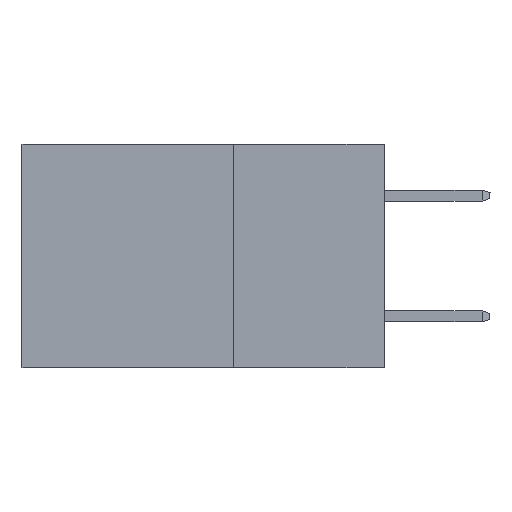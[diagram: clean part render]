
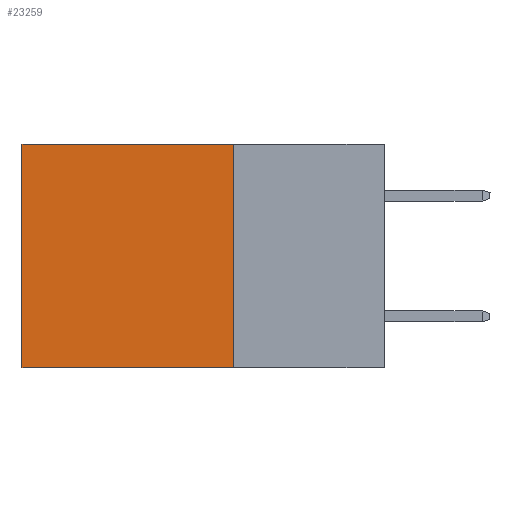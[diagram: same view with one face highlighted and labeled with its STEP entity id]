
A CAD part, left-side view. The second image highlights one B-rep face of the part: STEP entity #23259.
In plain terms, the highlighted planar face has unit normal (-1, 0, 0).
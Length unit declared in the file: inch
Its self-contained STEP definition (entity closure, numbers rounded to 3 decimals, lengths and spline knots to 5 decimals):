
#971 = DIRECTION ( 'NONE',  ( 0., 0., -1. ) ) ;
#2756 = LINE ( 'NONE', #4010, #26418 ) ;
#4010 = CARTESIAN_POINT ( 'NONE',  ( 0.298, 0.25, -0.37 ) ) ;
#5079 = LINE ( 'NONE', #21322, #25149 ) ;
#5418 = LINE ( 'NONE', #7522, #25087 ) ;
#7522 = CARTESIAN_POINT ( 'NONE',  ( 0.298, 0.6, 0. ) ) ;
#8998 = AXIS2_PLACEMENT_3D ( 'NONE', #10248, #12947, #971 ) ;
#9836 = CARTESIAN_POINT ( 'NONE',  ( 0.298, 0.6, 0. ) ) ;
#10248 = CARTESIAN_POINT ( 'NONE',  ( 0.298, 0.25, 0. ) ) ;
#10481 = FACE_OUTER_BOUND ( 'NONE', #30135, .T. ) ;
#11944 = ORIENTED_EDGE ( 'NONE', *, *, #13231, .F. ) ;
#12947 = DIRECTION ( 'NONE',  ( 1., 0., 0. ) ) ;
#13231 = EDGE_CURVE ( 'NONE', #31342, #13552, #5079, .T. ) ;
#13546 = CARTESIAN_POINT ( 'NONE',  ( 0.298, 0.25, -0.37 ) ) ;
#13552 = VERTEX_POINT ( 'NONE', #13546 ) ;
#17504 = CARTESIAN_POINT ( 'NONE',  ( 0.298, 0.25, 0. ) ) ;
#18831 = DIRECTION ( 'NONE',  ( 0., 0., -1. ) ) ;
#19701 = ORIENTED_EDGE ( 'NONE', *, *, #27869, .T. ) ;
#20263 = ORIENTED_EDGE ( 'NONE', *, *, #33011, .F. ) ;
#20849 = DIRECTION ( 'NONE',  ( 0., 1., 0. ) ) ;
#20866 = VECTOR ( 'NONE', #25753, 39.37008 ) ;
#20889 = CARTESIAN_POINT ( 'NONE',  ( 0.298, 0.25, 0. ) ) ;
#21322 = CARTESIAN_POINT ( 'NONE',  ( 0.298, 0.25, 0. ) ) ;
#22076 = LINE ( 'NONE', #20889, #20866 ) ;
#22789 = DIRECTION ( 'NONE',  ( 0., 0., -1. ) ) ;
#22972 = PLANE ( 'NONE',  #8998 ) ;
#23259 = ADVANCED_FACE ( 'NONE', ( #10481 ), #22972, .F. ) ;
#24257 = EDGE_CURVE ( 'NONE', #31342, #25767, #22076, .T. ) ;
#24762 = ORIENTED_EDGE ( 'NONE', *, *, #24257, .T. ) ;
#25087 = VECTOR ( 'NONE', #22789, 39.37008 ) ;
#25149 = VECTOR ( 'NONE', #18831, 39.37008 ) ;
#25462 = CARTESIAN_POINT ( 'NONE',  ( 0.298, 0.6, -0.37 ) ) ;
#25753 = DIRECTION ( 'NONE',  ( 0., 1., 0. ) ) ;
#25767 = VERTEX_POINT ( 'NONE', #9836 ) ;
#26343 = VERTEX_POINT ( 'NONE', #25462 ) ;
#26418 = VECTOR ( 'NONE', #20849, 39.37008 ) ;
#27869 = EDGE_CURVE ( 'NONE', #25767, #26343, #5418, .T. ) ;
#30135 = EDGE_LOOP ( 'NONE', ( #19701, #20263, #11944, #24762 ) ) ;
#31342 = VERTEX_POINT ( 'NONE', #17504 ) ;
#33011 = EDGE_CURVE ( 'NONE', #13552, #26343, #2756, .T. ) ;
